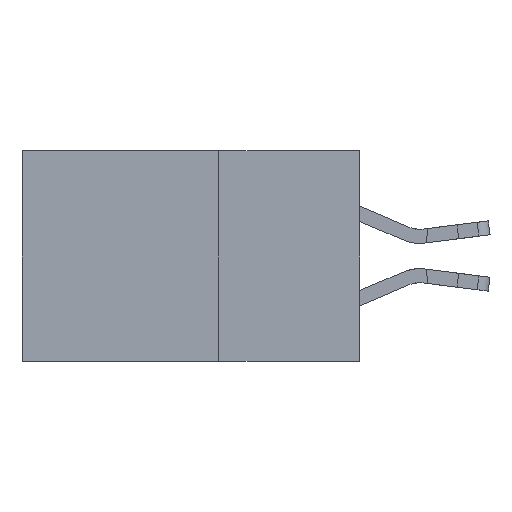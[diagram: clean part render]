
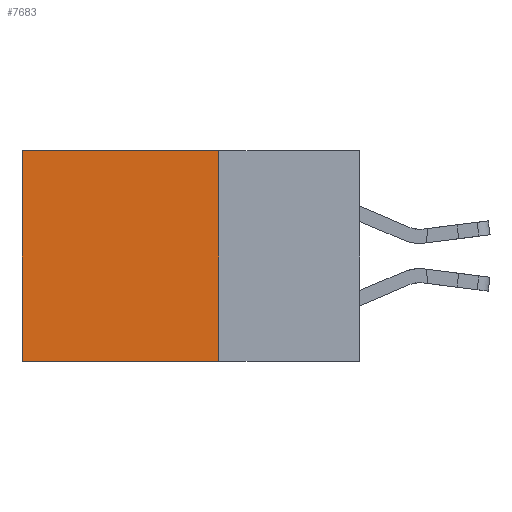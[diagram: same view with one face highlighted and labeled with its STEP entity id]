
A CAD part, left-side view. The second image highlights one B-rep face of the part: STEP entity #7683.
In plain terms, the highlighted planar face has unit normal (-1, 0, 0).
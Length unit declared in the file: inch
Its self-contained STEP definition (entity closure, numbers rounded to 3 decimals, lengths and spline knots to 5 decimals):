
#51 = VERTEX_POINT ( 'NONE', #5943 ) ;
#273 = LINE ( 'NONE', #3785, #14626 ) ;
#354 = PLANE ( 'NONE',  #3064 ) ;
#392 = CARTESIAN_POINT ( 'NONE',  ( 0.2875, 0.25, -0.375 ) ) ;
#538 = EDGE_CURVE ( 'NONE', #51, #14355, #7135, .T. ) ;
#1108 = VECTOR ( 'NONE', #5537, 39.37008 ) ;
#1604 = CARTESIAN_POINT ( 'NONE',  ( 0.2875, 0.25, -0.375 ) ) ;
#1819 = EDGE_CURVE ( 'NONE', #51, #13347, #7662, .T. ) ;
#1871 = DIRECTION ( 'NONE',  ( 0., 0., -1. ) ) ;
#1959 = CARTESIAN_POINT ( 'NONE',  ( 0.2875, 0.25, 0. ) ) ;
#2573 = FACE_OUTER_BOUND ( 'NONE', #7622, .T. ) ;
#2898 = ORIENTED_EDGE ( 'NONE', *, *, #1819, .F. ) ;
#3064 = AXIS2_PLACEMENT_3D ( 'NONE', #1604, #4291, #1871 ) ;
#3298 = CARTESIAN_POINT ( 'NONE',  ( 0.2875, 0.6, -0.375 ) ) ;
#3785 = CARTESIAN_POINT ( 'NONE',  ( 0.2875, 0.6, -0.375 ) ) ;
#3962 = VECTOR ( 'NONE', #9893, 39.37008 ) ;
#4291 = DIRECTION ( 'NONE',  ( 1., 0., 0. ) ) ;
#5037 = CARTESIAN_POINT ( 'NONE',  ( 0.2875, 0.6, 0. ) ) ;
#5537 = DIRECTION ( 'NONE',  ( 0., 1., 0. ) ) ;
#5722 = EDGE_CURVE ( 'NONE', #13347, #8382, #8233, .T. ) ;
#5943 = CARTESIAN_POINT ( 'NONE',  ( 0.2875, 0.25, 0. ) ) ;
#6355 = ORIENTED_EDGE ( 'NONE', *, *, #5722, .F. ) ;
#7135 = LINE ( 'NONE', #1959, #1108 ) ;
#7590 = DIRECTION ( 'NONE',  ( 0., 0., -1. ) ) ;
#7622 = EDGE_LOOP ( 'NONE', ( #10618, #6355, #2898, #12067 ) ) ;
#7662 = LINE ( 'NONE', #12342, #3962 ) ;
#7683 = ADVANCED_FACE ( 'NONE', ( #2573 ), #354, .F. ) ;
#8233 = LINE ( 'NONE', #13594, #15012 ) ;
#8382 = VERTEX_POINT ( 'NONE', #3298 ) ;
#9893 = DIRECTION ( 'NONE',  ( 0., 0., -1. ) ) ;
#10618 = ORIENTED_EDGE ( 'NONE', *, *, #15263, .T. ) ;
#12067 = ORIENTED_EDGE ( 'NONE', *, *, #538, .T. ) ;
#12271 = DIRECTION ( 'NONE',  ( 0., 1., 0. ) ) ;
#12342 = CARTESIAN_POINT ( 'NONE',  ( 0.2875, 0.25, -0.375 ) ) ;
#13347 = VERTEX_POINT ( 'NONE', #392 ) ;
#13594 = CARTESIAN_POINT ( 'NONE',  ( 0.2875, 0.25, -0.375 ) ) ;
#14355 = VERTEX_POINT ( 'NONE', #5037 ) ;
#14626 = VECTOR ( 'NONE', #7590, 39.37008 ) ;
#15012 = VECTOR ( 'NONE', #12271, 39.37008 ) ;
#15263 = EDGE_CURVE ( 'NONE', #14355, #8382, #273, .T. ) ;
